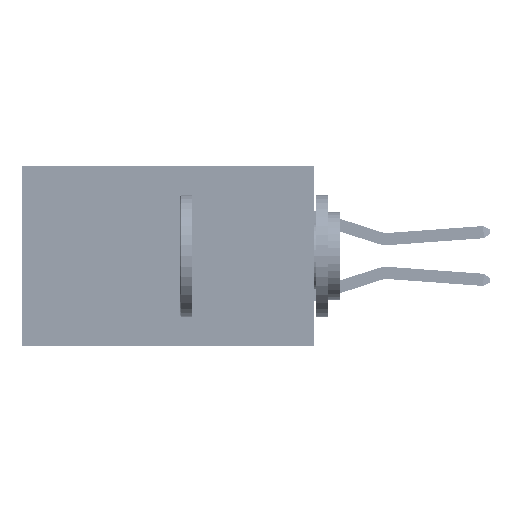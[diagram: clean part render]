
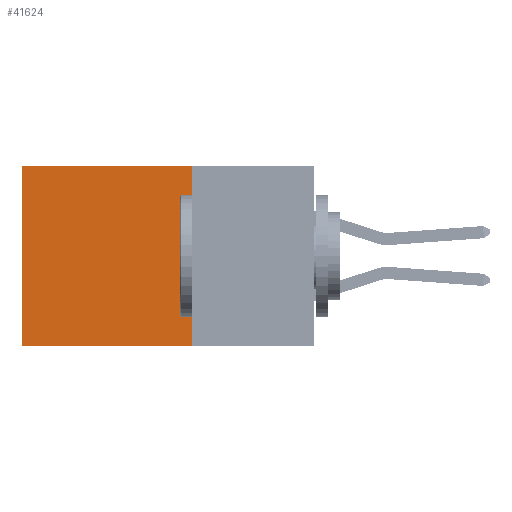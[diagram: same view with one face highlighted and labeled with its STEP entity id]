
A CAD part, left-side view. The second image highlights one B-rep face of the part: STEP entity #41624.
In plain terms, the highlighted planar face has unit normal (-1, 0, 0).
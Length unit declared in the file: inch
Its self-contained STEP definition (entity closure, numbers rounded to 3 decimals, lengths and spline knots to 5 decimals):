
#1009 = LINE ( 'NONE', #2265, #49281 ) ;
#1345 = VERTEX_POINT ( 'NONE', #21412 ) ;
#2084 = DIRECTION ( 'NONE',  ( 0., 1., 0. ) ) ;
#2257 = CARTESIAN_POINT ( 'NONE',  ( 0.2875, 0.6, 0. ) ) ;
#2265 = CARTESIAN_POINT ( 'NONE',  ( 0.2875, 0.25, 0. ) ) ;
#2333 = LINE ( 'NONE', #17542, #42555 ) ;
#3686 = CARTESIAN_POINT ( 'NONE',  ( 0.2875, 0.25, -0.37 ) ) ;
#5316 = EDGE_CURVE ( 'NONE', #14178, #21098, #2333, .T. ) ;
#6196 = EDGE_CURVE ( 'NONE', #39056, #21098, #37478, .T. ) ;
#6387 = ORIENTED_EDGE ( 'NONE', *, *, #5316, .F. ) ;
#7535 = PLANE ( 'NONE',  #10665 ) ;
#10604 = EDGE_CURVE ( 'NONE', #1345, #39056, #1009, .T. ) ;
#10665 = AXIS2_PLACEMENT_3D ( 'NONE', #11528, #42669, #23303 ) ;
#11528 = CARTESIAN_POINT ( 'NONE',  ( 0.2875, 0.25, 0. ) ) ;
#14178 = VERTEX_POINT ( 'NONE', #3686 ) ;
#17542 = CARTESIAN_POINT ( 'NONE',  ( 0.2875, 0.25, -0.37 ) ) ;
#18846 = LINE ( 'NONE', #21604, #38617 ) ;
#19598 = VECTOR ( 'NONE', #26331, 39.37008 ) ;
#21098 = VERTEX_POINT ( 'NONE', #44864 ) ;
#21412 = CARTESIAN_POINT ( 'NONE',  ( 0.2875, 0.25, 0. ) ) ;
#21604 = CARTESIAN_POINT ( 'NONE',  ( 0.2875, 0.25, 0. ) ) ;
#21722 = DIRECTION ( 'NONE',  ( 0., 1., 0. ) ) ;
#23303 = DIRECTION ( 'NONE',  ( 0., 0., -1. ) ) ;
#23761 = FACE_OUTER_BOUND ( 'NONE', #35902, .T. ) ;
#25562 = DIRECTION ( 'NONE',  ( 0., 0., -1. ) ) ;
#26331 = DIRECTION ( 'NONE',  ( 0., 0., -1. ) ) ;
#27056 = ORIENTED_EDGE ( 'NONE', *, *, #6196, .T. ) ;
#27788 = ORIENTED_EDGE ( 'NONE', *, *, #10604, .T. ) ;
#28350 = ORIENTED_EDGE ( 'NONE', *, *, #29053, .F. ) ;
#29053 = EDGE_CURVE ( 'NONE', #1345, #14178, #18846, .T. ) ;
#31757 = CARTESIAN_POINT ( 'NONE',  ( 0.2875, 0.6, 0. ) ) ;
#35902 = EDGE_LOOP ( 'NONE', ( #27056, #6387, #28350, #27788 ) ) ;
#37478 = LINE ( 'NONE', #2257, #19598 ) ;
#38617 = VECTOR ( 'NONE', #25562, 39.37008 ) ;
#39056 = VERTEX_POINT ( 'NONE', #31757 ) ;
#41624 = ADVANCED_FACE ( 'NONE', ( #23761 ), #7535, .F. ) ;
#42555 = VECTOR ( 'NONE', #21722, 39.37008 ) ;
#42669 = DIRECTION ( 'NONE',  ( 1., 0., 0. ) ) ;
#44864 = CARTESIAN_POINT ( 'NONE',  ( 0.2875, 0.6, -0.37 ) ) ;
#49281 = VECTOR ( 'NONE', #2084, 39.37008 ) ;
